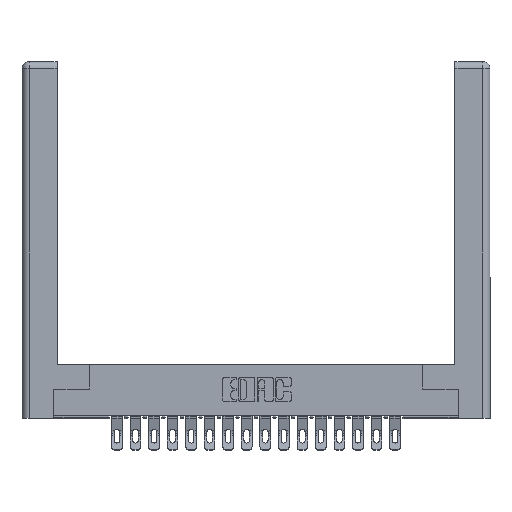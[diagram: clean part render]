
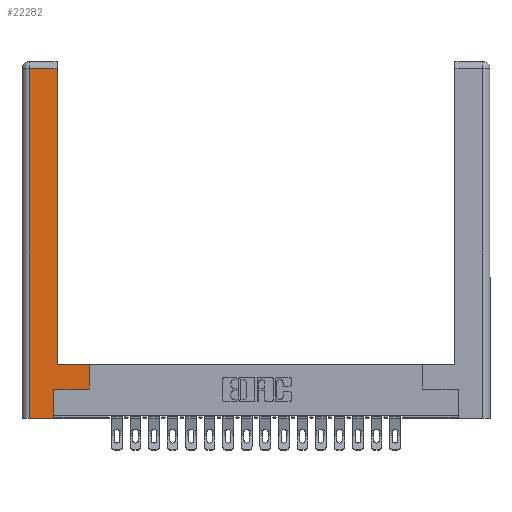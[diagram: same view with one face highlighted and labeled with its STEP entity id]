
A CAD part, top view. The second image highlights one B-rep face of the part: STEP entity #22282.
In plain terms, the highlighted planar face has unit normal (0, 0, 1).
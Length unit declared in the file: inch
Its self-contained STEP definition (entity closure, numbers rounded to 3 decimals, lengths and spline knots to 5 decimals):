
#167 = VECTOR ( 'NONE', #7313, 39.37008 ) ;
#1306 = EDGE_CURVE ( 'NONE', #21240, #19678, #18919, .T. ) ;
#1884 = VERTEX_POINT ( 'NONE', #3531 ) ;
#2276 = EDGE_CURVE ( 'NONE', #20450, #22543, #12303, .T. ) ;
#2920 = VERTEX_POINT ( 'NONE', #11020 ) ;
#3126 = LINE ( 'NONE', #21755, #13174 ) ;
#3243 = CARTESIAN_POINT ( 'NONE',  ( 0.565, 0.245, 0. ) ) ;
#3531 = CARTESIAN_POINT ( 'NONE',  ( 0.265, 0.245, 0. ) ) ;
#3761 = AXIS2_PLACEMENT_3D ( 'NONE', #11757, #4480, #19142 ) ;
#3958 = CARTESIAN_POINT ( 'NONE',  ( 0.0615, 2.94, 0. ) ) ;
#4166 = ORIENTED_EDGE ( 'NONE', *, *, #1306, .T. ) ;
#4480 = DIRECTION ( 'NONE',  ( 0., 0., -1. ) ) ;
#5264 = EDGE_CURVE ( 'NONE', #7987, #20450, #7729, .T. ) ;
#5828 = FACE_OUTER_BOUND ( 'NONE', #18305, .T. ) ;
#6560 = CARTESIAN_POINT ( 'NONE',  ( 0.565, 0.45, 0. ) ) ;
#7313 = DIRECTION ( 'NONE',  ( 1., 0., 0. ) ) ;
#7481 = CARTESIAN_POINT ( 'NONE',  ( 0.295, 2.94, 0. ) ) ;
#7729 = LINE ( 'NONE', #18731, #21679 ) ;
#7987 = VERTEX_POINT ( 'NONE', #8679 ) ;
#8006 = DIRECTION ( 'NONE',  ( 0., -1., 0. ) ) ;
#8277 = LINE ( 'NONE', #10971, #167 ) ;
#8679 = CARTESIAN_POINT ( 'NONE',  ( 0.295, 0.45, 0. ) ) ;
#9325 = EDGE_CURVE ( 'NONE', #2920, #11378, #8277, .T. ) ;
#9680 = CARTESIAN_POINT ( 'NONE',  ( 0.0615, 2.94, 0. ) ) ;
#10728 = ORIENTED_EDGE ( 'NONE', *, *, #9325, .T. ) ;
#10971 = CARTESIAN_POINT ( 'NONE',  ( 0.265, 0., 0. ) ) ;
#11020 = CARTESIAN_POINT ( 'NONE',  ( 0.0615, 0., 0. ) ) ;
#11378 = VERTEX_POINT ( 'NONE', #21733 ) ;
#11413 = ORIENTED_EDGE ( 'NONE', *, *, #17105, .T. ) ;
#11757 = CARTESIAN_POINT ( 'NONE',  ( 0., 0., 0. ) ) ;
#11789 = VECTOR ( 'NONE', #8006, 39.37008 ) ;
#12037 = VECTOR ( 'NONE', #20735, 39.37008 ) ;
#12204 = DIRECTION ( 'NONE',  ( -1., 0., 0. ) ) ;
#12303 = LINE ( 'NONE', #9680, #12037 ) ;
#12367 = VECTOR ( 'NONE', #19132, 39.37008 ) ;
#12642 = DIRECTION ( 'NONE',  ( 1., 0., 0. ) ) ;
#12948 = CARTESIAN_POINT ( 'NONE',  ( 0.265, 0.245, 0. ) ) ;
#12961 = CARTESIAN_POINT ( 'NONE',  ( 0.565, 0.45, 0. ) ) ;
#13174 = VECTOR ( 'NONE', #12642, 39.37008 ) ;
#13488 = EDGE_CURVE ( 'NONE', #11378, #1884, #18615, .T. ) ;
#13982 = ORIENTED_EDGE ( 'NONE', *, *, #14589, .T. ) ;
#14094 = CARTESIAN_POINT ( 'NONE',  ( 0.295, 0.45, 0. ) ) ;
#14589 = EDGE_CURVE ( 'NONE', #1884, #21240, #3126, .T. ) ;
#14820 = ORIENTED_EDGE ( 'NONE', *, *, #13488, .T. ) ;
#15013 = ORIENTED_EDGE ( 'NONE', *, *, #18955, .T. ) ;
#15153 = DIRECTION ( 'NONE',  ( 0., 1., 0. ) ) ;
#15391 = PLANE ( 'NONE',  #3761 ) ;
#16606 = LINE ( 'NONE', #22598, #11789 ) ;
#16940 = LINE ( 'NONE', #14094, #18663 ) ;
#17105 = EDGE_CURVE ( 'NONE', #19678, #7987, #16940, .T. ) ;
#17727 = ORIENTED_EDGE ( 'NONE', *, *, #2276, .T. ) ;
#18305 = EDGE_LOOP ( 'NONE', ( #22159, #17727, #15013, #10728, #14820, #13982, #4166, #11413 ) ) ;
#18615 = LINE ( 'NONE', #12948, #21773 ) ;
#18663 = VECTOR ( 'NONE', #12204, 39.37008 ) ;
#18731 = CARTESIAN_POINT ( 'NONE',  ( 0.295, 3., 0. ) ) ;
#18919 = LINE ( 'NONE', #6560, #12367 ) ;
#18955 = EDGE_CURVE ( 'NONE', #22543, #2920, #16606, .T. ) ;
#19132 = DIRECTION ( 'NONE',  ( 0., 1., 0. ) ) ;
#19142 = DIRECTION ( 'NONE',  ( -1., 0., 0. ) ) ;
#19678 = VERTEX_POINT ( 'NONE', #12961 ) ;
#20450 = VERTEX_POINT ( 'NONE', #7481 ) ;
#20735 = DIRECTION ( 'NONE',  ( -1., 0., 0. ) ) ;
#21240 = VERTEX_POINT ( 'NONE', #3243 ) ;
#21679 = VECTOR ( 'NONE', #15153, 39.37008 ) ;
#21733 = CARTESIAN_POINT ( 'NONE',  ( 0.265, 0., 0. ) ) ;
#21755 = CARTESIAN_POINT ( 'NONE',  ( 0.565, 0.245, 0. ) ) ;
#21773 = VECTOR ( 'NONE', #21820, 39.37008 ) ;
#21820 = DIRECTION ( 'NONE',  ( 0., 1., 0. ) ) ;
#22159 = ORIENTED_EDGE ( 'NONE', *, *, #5264, .T. ) ;
#22282 = ADVANCED_FACE ( 'NONE', ( #5828 ), #15391, .F. ) ;
#22543 = VERTEX_POINT ( 'NONE', #3958 ) ;
#22598 = CARTESIAN_POINT ( 'NONE',  ( 0.0615, 0., 0. ) ) ;
